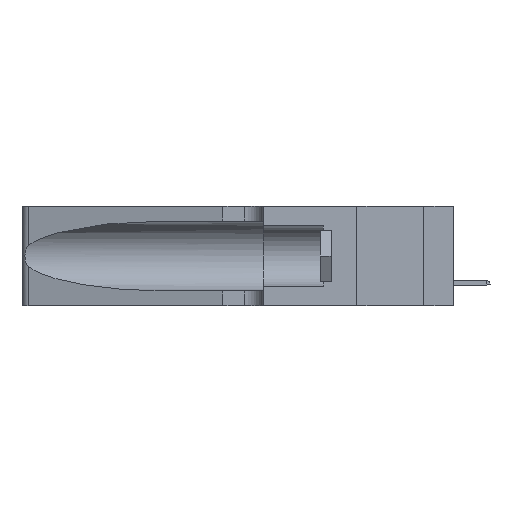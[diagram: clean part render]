
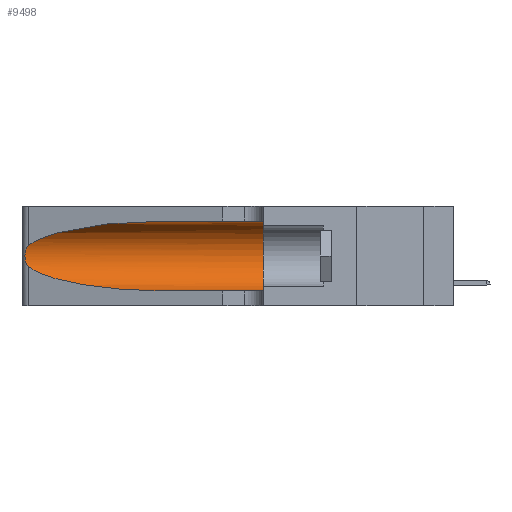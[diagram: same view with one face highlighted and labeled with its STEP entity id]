
A CAD part, left-side view. The second image highlights one B-rep face of the part: STEP entity #9498.
In plain terms, the highlighted cylindrical face has radius 3.308 mm (diameter 6.617 mm), a partial arc.
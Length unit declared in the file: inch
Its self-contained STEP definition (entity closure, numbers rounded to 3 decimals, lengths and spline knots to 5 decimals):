
#315 = CARTESIAN_POINT ( 'NONE',  ( 0.18966, 0.96281, 0.31525 ) ) ;
#1199 = CARTESIAN_POINT ( 'NONE',  ( 0.1305, 1.61858, 0.05475 ) ) ;
#1659 = ORIENTED_EDGE ( 'NONE', *, *, #10354, .T. ) ;
#1976 = CARTESIAN_POINT ( 'NONE',  ( 0.1305, 1.61858, 0.185 ) ) ;
#2906 = CARTESIAN_POINT ( 'NONE',  ( 0.25487, 1.22718, 0.22369 ) ) ;
#3937 = DIRECTION ( 'NONE',  ( 0., 1., 0. ) ) ;
#3983 = CYLINDRICAL_SURFACE ( 'NONE', #23178, 0.13025 ) ;
#4082 = ORIENTED_EDGE ( 'NONE', *, *, #6246, .T. ) ;
#4658 = CARTESIAN_POINT ( 'NONE',  ( 0.26075, 1.23896, 0.19203 ) ) ;
#4911 = CARTESIAN_POINT ( 'NONE',  ( 0.26075, 1.23896, 0.178 ) ) ;
#4941 = VERTEX_POINT ( 'NONE', #14136 ) ;
#5757 = FACE_OUTER_BOUND ( 'NONE', #22502, .T. ) ;
#6081 = CARTESIAN_POINT ( 'NONE',  ( 0.18966, 0.96281, 0.05475 ) ) ;
#6199 =( BOUNDED_CURVE ( )  B_SPLINE_CURVE ( 3, ( #13686, #22803, #6081, #19435 ),
 .UNSPECIFIED., .F., .F. ) 
 B_SPLINE_CURVE_WITH_KNOTS ( ( 4, 4 ),
 ( 3.44316, 4.71239 ),
 .UNSPECIFIED. ) 
 CURVE ( )  GEOMETRIC_REPRESENTATION_ITEM ( )  RATIONAL_B_SPLINE_CURVE ( ( 1., 0.87, 0.87, 1. ) ) 
 REPRESENTATION_ITEM ( '' )  );
#6246 = EDGE_CURVE ( 'NONE', #22858, #10481, #20336, .T. ) ;
#6359 = CARTESIAN_POINT ( 'NONE',  ( 0.25487, 1.22718, 0.22369 ) ) ;
#6531 = VERTEX_POINT ( 'NONE', #21089 ) ;
#6702 = CARTESIAN_POINT ( 'NONE',  ( 0.25487, 1.22718, 0.14631 ) ) ;
#8653 = EDGE_CURVE ( 'NONE', #10481, #4941, #6199, .T. ) ;
#9494 = DIRECTION ( 'NONE',  ( 0., 0., 1. ) ) ;
#9498 = ADVANCED_FACE ( 'NONE', ( #5757 ), #3983, .F. ) ;
#9506 = CARTESIAN_POINT ( 'NONE',  ( 0.1305, 0.72297, 0.31525 ) ) ;
#9962 = ORIENTED_EDGE ( 'NONE', *, *, #18211, .F. ) ;
#10081 = VERTEX_POINT ( 'NONE', #13478 ) ;
#10354 = EDGE_CURVE ( 'NONE', #4941, #10081, #18334, .T. ) ;
#10481 = VERTEX_POINT ( 'NONE', #11472 ) ;
#10815 = CARTESIAN_POINT ( 'NONE',  ( 0.25789, 1.23486, 0.15765 ) ) ;
#11464 = CARTESIAN_POINT ( 'NONE',  ( 0.1305, 1.61858, 0.31525 ) ) ;
#11472 = CARTESIAN_POINT ( 'NONE',  ( 0.25487, 1.22718, 0.14631 ) ) ;
#11494 = CARTESIAN_POINT ( 'NONE',  ( 0.1305, 0.72297, 0.31525 ) ) ;
#11984 = CARTESIAN_POINT ( 'NONE',  ( 0.26018, 1.23835, 0.19895 ) ) ;
#12694 = ORIENTED_EDGE ( 'NONE', *, *, #8653, .T. ) ;
#13478 = CARTESIAN_POINT ( 'NONE',  ( 0.1305, 0.35, 0.05475 ) ) ;
#13535 = EDGE_CURVE ( 'NONE', #6531, #10081, #13760, .T. ) ;
#13620 = DIRECTION ( 'NONE',  ( 0., -1., 0. ) ) ;
#13686 = CARTESIAN_POINT ( 'NONE',  ( 0.25487, 1.22718, 0.14631 ) ) ;
#13760 = CIRCLE ( 'NONE', #20514, 0.13025 ) ;
#14136 = CARTESIAN_POINT ( 'NONE',  ( 0.1305, 0.72297, 0.05475 ) ) ;
#14428 = VECTOR ( 'NONE', #24083, 39.37008 ) ;
#15845 = VECTOR ( 'NONE', #24564, 39.37008 ) ;
#15934 = CARTESIAN_POINT ( 'NONE',  ( 0.25639, 1.23184, 0.21858 ) ) ;
#17339 = ORIENTED_EDGE ( 'NONE', *, *, #13535, .F. ) ;
#17424 = LINE ( 'NONE', #11464, #15845 ) ;
#17936 = CARTESIAN_POINT ( 'NONE',  ( 0.25854, 1.2359, 0.20912 ) ) ;
#17976 = ORIENTED_EDGE ( 'NONE', *, *, #22152, .T. ) ;
#18211 = EDGE_CURVE ( 'NONE', #23818, #6531, #17424, .T. ) ;
#18334 = LINE ( 'NONE', #1199, #14428 ) ;
#18398 = CARTESIAN_POINT ( 'NONE',  ( 0.25639, 1.23186, 0.15144 ) ) ;
#18824 = CARTESIAN_POINT ( 'NONE',  ( 0.2373, 1.15595, 0.28018 ) ) ;
#19072 = CARTESIAN_POINT ( 'NONE',  ( 0.25487, 1.22718, 0.22369 ) ) ;
#19435 = CARTESIAN_POINT ( 'NONE',  ( 0.1305, 0.72297, 0.05475 ) ) ;
#19895 = CARTESIAN_POINT ( 'NONE',  ( 0.25555, 1.22993, 0.14849 ) ) ;
#20133 = CARTESIAN_POINT ( 'NONE',  ( 0.25856, 1.23593, 0.16098 ) ) ;
#20336 = B_SPLINE_CURVE_WITH_KNOTS ( 'NONE', 3,
 ( #6359, #21559, #15934, #21445, #17936, #11984, #4658, #4911, #21770, #20133, #10815, #18398, #19895, #6702 ),
 .UNSPECIFIED., .F., .F.,
 ( 4, 2, 2, 2, 2, 2, 4 ),
 ( 0., 0.00027, 0.00053, 0.00107, 0.0016, 0.00187, 0.00214 ),
 .UNSPECIFIED. ) ;
#20514 = AXIS2_PLACEMENT_3D ( 'NONE', #21180, #3937, #9494 ) ;
#21089 = CARTESIAN_POINT ( 'NONE',  ( 0.1305, 0.35, 0.31525 ) ) ;
#21180 = CARTESIAN_POINT ( 'NONE',  ( 0.1305, 0.35, 0.185 ) ) ;
#21445 = CARTESIAN_POINT ( 'NONE',  ( 0.25787, 1.23484, 0.2124 ) ) ;
#21559 = CARTESIAN_POINT ( 'NONE',  ( 0.25555, 1.22994, 0.2215 ) ) ;
#21770 = CARTESIAN_POINT ( 'NONE',  ( 0.26017, 1.23833, 0.17102 ) ) ;
#22152 = EDGE_CURVE ( 'NONE', #23818, #22858, #23236, .T. ) ;
#22502 = EDGE_LOOP ( 'NONE', ( #17976, #4082, #12694, #1659, #17339, #9962 ) ) ;
#22803 = CARTESIAN_POINT ( 'NONE',  ( 0.2373, 1.15595, 0.08982 ) ) ;
#22858 = VERTEX_POINT ( 'NONE', #2906 ) ;
#23178 = AXIS2_PLACEMENT_3D ( 'NONE', #1976, #13620, #24500 ) ;
#23236 =( BOUNDED_CURVE ( )  B_SPLINE_CURVE ( 3, ( #11494, #315, #18824, #19072 ),
 .UNSPECIFIED., .F., .F. ) 
 B_SPLINE_CURVE_WITH_KNOTS ( ( 4, 4 ),
 ( 1.5708, 2.84003 ),
 .UNSPECIFIED. ) 
 CURVE ( )  GEOMETRIC_REPRESENTATION_ITEM ( )  RATIONAL_B_SPLINE_CURVE ( ( 1., 0.87, 0.87, 1. ) ) 
 REPRESENTATION_ITEM ( '' )  );
#23818 = VERTEX_POINT ( 'NONE', #9506 ) ;
#24083 = DIRECTION ( 'NONE',  ( 0., -1., 0. ) ) ;
#24500 = DIRECTION ( 'NONE',  ( 0., 0., -1. ) ) ;
#24564 = DIRECTION ( 'NONE',  ( 0., -1., 0. ) ) ;
